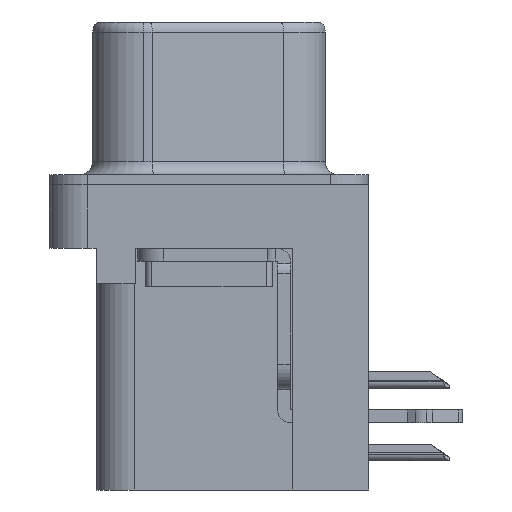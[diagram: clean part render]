
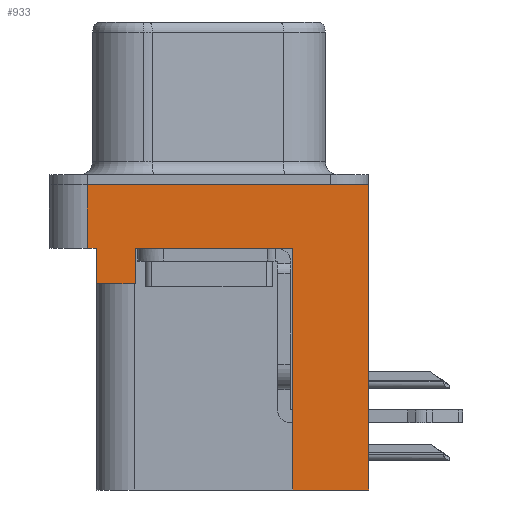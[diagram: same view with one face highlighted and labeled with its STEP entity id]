
A CAD part, left-side view. The second image highlights one B-rep face of the part: STEP entity #933.
In plain terms, the highlighted planar face has unit normal (-1, 0, 0).
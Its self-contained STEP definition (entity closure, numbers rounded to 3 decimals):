
#315 = DIRECTION ( 'NONE',  ( 0., 1., 0. ) ) ;
#559 = VECTOR ( 'NONE', #14995, 1000. ) ;
#680 = DIRECTION ( 'NONE',  ( 0., 0., 1. ) ) ;
#933 = ADVANCED_FACE ( 'NONE', ( #5806 ), #14279, .T. ) ;
#1084 = EDGE_CURVE ( 'NONE', #10015, #13459, #3467, .T. ) ;
#1185 = VECTOR ( 'NONE', #15367, 1000. ) ;
#1704 = DIRECTION ( 'NONE',  ( 0., -1., 0. ) ) ;
#1990 = LINE ( 'NONE', #19319, #11199 ) ;
#2221 = CARTESIAN_POINT ( 'NONE',  ( -2.91, 4.425, -3.9 ) ) ;
#2251 = VERTEX_POINT ( 'NONE', #13994 ) ;
#2427 = EDGE_CURVE ( 'NONE', #27087, #23379, #9965, .T. ) ;
#2591 = DIRECTION ( 'NONE',  ( 0., 0., 1. ) ) ;
#3096 = ORIENTED_EDGE ( 'NONE', *, *, #17878, .F. ) ;
#3099 = CARTESIAN_POINT ( 'NONE',  ( -2.91, -6.275, -2.5 ) ) ;
#3270 = EDGE_CURVE ( 'NONE', #14589, #13638, #17617, .T. ) ;
#3467 = LINE ( 'NONE', #3099, #11939 ) ;
#3615 = CARTESIAN_POINT ( 'NONE',  ( -2.91, 4.775, -2.5 ) ) ;
#4461 = DIRECTION ( 'NONE',  ( 0., 0., 1. ) ) ;
#4589 = CARTESIAN_POINT ( 'NONE',  ( -2.91, 2.895, -3.9 ) ) ;
#5471 = VECTOR ( 'NONE', #4461, 1000. ) ;
#5806 = FACE_OUTER_BOUND ( 'NONE', #22353, .T. ) ;
#6202 = DIRECTION ( 'NONE',  ( 0., 0., 1. ) ) ;
#6781 = CARTESIAN_POINT ( 'NONE',  ( -2.91, 4.775, -2.5 ) ) ;
#6959 = EDGE_CURVE ( 'NONE', #27087, #10015, #1990, .T. ) ;
#8123 = EDGE_CURVE ( 'NONE', #10160, #13638, #23810, .T. ) ;
#8305 = ORIENTED_EDGE ( 'NONE', *, *, #1084, .T. ) ;
#8805 = VECTOR ( 'NONE', #23846, 1000. ) ;
#9011 = CARTESIAN_POINT ( 'NONE',  ( -2.91, 4.775, 0. ) ) ;
#9449 = LINE ( 'NONE', #6781, #8805 ) ;
#9497 = CARTESIAN_POINT ( 'NONE',  ( -2.91, 4.425, -3.9 ) ) ;
#9588 = CARTESIAN_POINT ( 'NONE',  ( -2.91, -3.295, -12. ) ) ;
#9835 = CARTESIAN_POINT ( 'NONE',  ( -2.91, 4.425, -2.5 ) ) ;
#9953 = AXIS2_PLACEMENT_3D ( 'NONE', #24637, #20991, #6202 ) ;
#9965 = LINE ( 'NONE', #2221, #18058 ) ;
#10015 = VERTEX_POINT ( 'NONE', #12165 ) ;
#10028 = ORIENTED_EDGE ( 'NONE', *, *, #16734, .F. ) ;
#10160 = VERTEX_POINT ( 'NONE', #18010 ) ;
#10305 = CARTESIAN_POINT ( 'NONE',  ( -2.91, -6.275, -2.5 ) ) ;
#10362 = VERTEX_POINT ( 'NONE', #9835 ) ;
#11159 = DIRECTION ( 'NONE',  ( 0., -1., 0. ) ) ;
#11199 = VECTOR ( 'NONE', #2591, 1000. ) ;
#11917 = ORIENTED_EDGE ( 'NONE', *, *, #14576, .F. ) ;
#11939 = VECTOR ( 'NONE', #11159, 1000. ) ;
#12165 = CARTESIAN_POINT ( 'NONE',  ( -2.91, 2.895, -2.5 ) ) ;
#13459 = VERTEX_POINT ( 'NONE', #26215 ) ;
#13638 = VERTEX_POINT ( 'NONE', #15419 ) ;
#13994 = CARTESIAN_POINT ( 'NONE',  ( -2.91, -3.295, -12. ) ) ;
#14279 = PLANE ( 'NONE',  #9953 ) ;
#14480 = LINE ( 'NONE', #9588, #20967 ) ;
#14576 = EDGE_CURVE ( 'NONE', #2251, #13459, #14880, .T. ) ;
#14589 = VERTEX_POINT ( 'NONE', #9011 ) ;
#14740 = VERTEX_POINT ( 'NONE', #3615 ) ;
#14841 = ORIENTED_EDGE ( 'NONE', *, *, #8123, .T. ) ;
#14880 = LINE ( 'NONE', #23915, #5471 ) ;
#14995 = DIRECTION ( 'NONE',  ( 0., 0., 1. ) ) ;
#15367 = DIRECTION ( 'NONE',  ( 0., -1., 0. ) ) ;
#15419 = CARTESIAN_POINT ( 'NONE',  ( -2.91, -6.275, 0. ) ) ;
#16148 = ORIENTED_EDGE ( 'NONE', *, *, #3270, .F. ) ;
#16552 = ORIENTED_EDGE ( 'NONE', *, *, #2427, .F. ) ;
#16662 = ORIENTED_EDGE ( 'NONE', *, *, #21464, .T. ) ;
#16734 = EDGE_CURVE ( 'NONE', #23379, #10362, #26805, .T. ) ;
#17155 = CARTESIAN_POINT ( 'NONE',  ( -2.91, -6.275, -2.5 ) ) ;
#17360 = CARTESIAN_POINT ( 'NONE',  ( -2.91, -6.275, 0. ) ) ;
#17617 = LINE ( 'NONE', #17360, #1185 ) ;
#17878 = EDGE_CURVE ( 'NONE', #14740, #14589, #9449, .T. ) ;
#18010 = CARTESIAN_POINT ( 'NONE',  ( -2.91, -6.275, -12. ) ) ;
#18058 = VECTOR ( 'NONE', #315, 1000. ) ;
#18216 = LINE ( 'NONE', #10305, #20172 ) ;
#18322 = ORIENTED_EDGE ( 'NONE', *, *, #19392, .F. ) ;
#19276 = VECTOR ( 'NONE', #680, 1000. ) ;
#19319 = CARTESIAN_POINT ( 'NONE',  ( -2.91, 2.895, -3.9 ) ) ;
#19392 = EDGE_CURVE ( 'NONE', #10160, #2251, #14480, .T. ) ;
#20172 = VECTOR ( 'NONE', #1704, 1000. ) ;
#20967 = VECTOR ( 'NONE', #24106, 1000. ) ;
#20991 = DIRECTION ( 'NONE',  ( -1., 0., 0. ) ) ;
#21464 = EDGE_CURVE ( 'NONE', #14740, #10362, #18216, .T. ) ;
#22353 = EDGE_LOOP ( 'NONE', ( #16148, #3096, #16662, #10028, #16552, #22481, #8305, #11917, #18322, #14841 ) ) ;
#22481 = ORIENTED_EDGE ( 'NONE', *, *, #6959, .T. ) ;
#23379 = VERTEX_POINT ( 'NONE', #23880 ) ;
#23810 = LINE ( 'NONE', #17155, #559 ) ;
#23846 = DIRECTION ( 'NONE',  ( 0., 0., 1. ) ) ;
#23880 = CARTESIAN_POINT ( 'NONE',  ( -2.91, 4.425, -3.9 ) ) ;
#23915 = CARTESIAN_POINT ( 'NONE',  ( -2.91, -3.295, -12. ) ) ;
#24106 = DIRECTION ( 'NONE',  ( 0., 1., 0. ) ) ;
#24637 = CARTESIAN_POINT ( 'NONE',  ( -2.91, -6.275, -2.5 ) ) ;
#26215 = CARTESIAN_POINT ( 'NONE',  ( -2.91, -3.295, -2.5 ) ) ;
#26805 = LINE ( 'NONE', #9497, #19276 ) ;
#27087 = VERTEX_POINT ( 'NONE', #4589 ) ;
